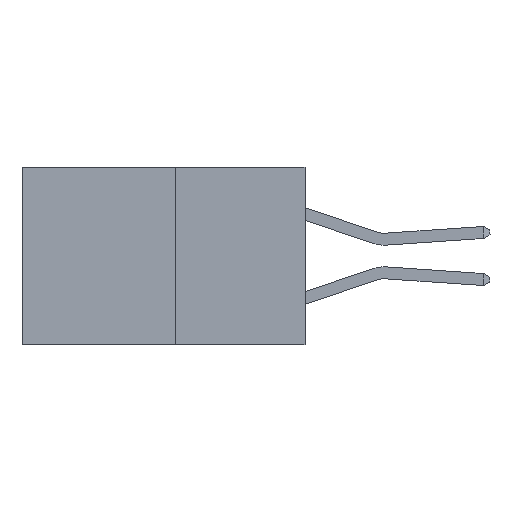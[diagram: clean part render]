
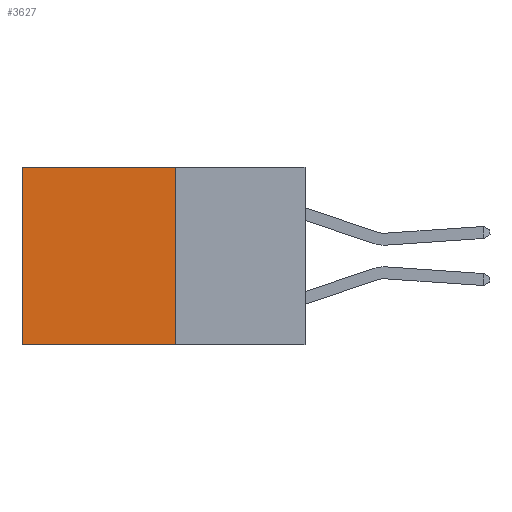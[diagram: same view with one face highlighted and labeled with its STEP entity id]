
A CAD part, left-side view. The second image highlights one B-rep face of the part: STEP entity #3627.
In plain terms, the highlighted planar face has unit normal (-1, 0, 0).
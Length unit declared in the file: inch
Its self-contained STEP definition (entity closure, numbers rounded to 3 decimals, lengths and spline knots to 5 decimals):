
#242 = EDGE_CURVE ( 'NONE', #673, #3495, #653, .T. ) ;
#614 = VECTOR ( 'NONE', #8794, 39.37008 ) ;
#653 = LINE ( 'NONE', #4514, #6515 ) ;
#673 = VERTEX_POINT ( 'NONE', #2007 ) ;
#882 = EDGE_CURVE ( 'NONE', #3495, #2669, #890, .T. ) ;
#890 = LINE ( 'NONE', #4168, #614 ) ;
#1552 = FACE_OUTER_BOUND ( 'NONE', #2080, .T. ) ;
#2007 = CARTESIAN_POINT ( 'NONE',  ( 0.277, 0.27, 0. ) ) ;
#2080 = EDGE_LOOP ( 'NONE', ( #3459, #6341, #2950, #3413 ) ) ;
#2273 = CARTESIAN_POINT ( 'NONE',  ( 0.277, 0.59, -0.37 ) ) ;
#2584 = CARTESIAN_POINT ( 'NONE',  ( 0.277, 0.27, 0. ) ) ;
#2661 = DIRECTION ( 'NONE',  ( 0., 1., 0. ) ) ;
#2669 = VERTEX_POINT ( 'NONE', #8835 ) ;
#2942 = CARTESIAN_POINT ( 'NONE',  ( 0.277, 0.27, -0.37 ) ) ;
#2950 = ORIENTED_EDGE ( 'NONE', *, *, #242, .F. ) ;
#3136 = DIRECTION ( 'NONE',  ( 0., 0., -1. ) ) ;
#3413 = ORIENTED_EDGE ( 'NONE', *, *, #4169, .T. ) ;
#3459 = ORIENTED_EDGE ( 'NONE', *, *, #7879, .T. ) ;
#3495 = VERTEX_POINT ( 'NONE', #2942 ) ;
#3627 = ADVANCED_FACE ( 'NONE', ( #1552 ), #9033, .F. ) ;
#3643 = VERTEX_POINT ( 'NONE', #8813 ) ;
#3870 = LINE ( 'NONE', #2273, #7506 ) ;
#4168 = CARTESIAN_POINT ( 'NONE',  ( 0.277, 0.27, -0.37 ) ) ;
#4169 = EDGE_CURVE ( 'NONE', #673, #3643, #7554, .T. ) ;
#4514 = CARTESIAN_POINT ( 'NONE',  ( 0.277, 0.27, -0.37 ) ) ;
#4987 = AXIS2_PLACEMENT_3D ( 'NONE', #9044, #9441, #9009 ) ;
#5713 = DIRECTION ( 'NONE',  ( 0., 0., -1. ) ) ;
#5910 = VECTOR ( 'NONE', #2661, 39.37008 ) ;
#6341 = ORIENTED_EDGE ( 'NONE', *, *, #882, .F. ) ;
#6515 = VECTOR ( 'NONE', #5713, 39.37008 ) ;
#7506 = VECTOR ( 'NONE', #3136, 39.37008 ) ;
#7554 = LINE ( 'NONE', #2584, #5910 ) ;
#7879 = EDGE_CURVE ( 'NONE', #3643, #2669, #3870, .T. ) ;
#8794 = DIRECTION ( 'NONE',  ( 0., 1., 0. ) ) ;
#8813 = CARTESIAN_POINT ( 'NONE',  ( 0.277, 0.59, 0. ) ) ;
#8835 = CARTESIAN_POINT ( 'NONE',  ( 0.277, 0.59, -0.37 ) ) ;
#9009 = DIRECTION ( 'NONE',  ( 0., 0., -1. ) ) ;
#9033 = PLANE ( 'NONE',  #4987 ) ;
#9044 = CARTESIAN_POINT ( 'NONE',  ( 0.277, 0.27, -0.37 ) ) ;
#9441 = DIRECTION ( 'NONE',  ( 1., 0., 0. ) ) ;
